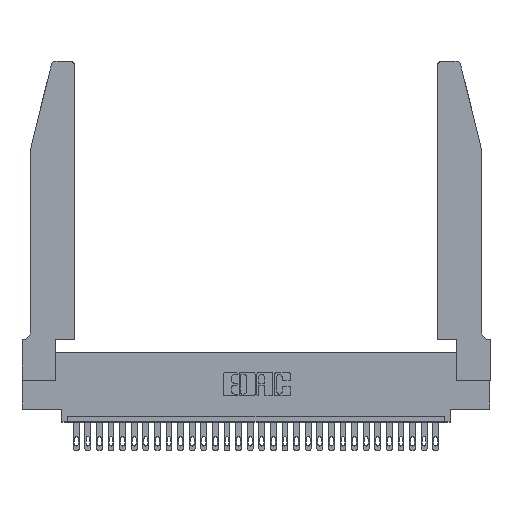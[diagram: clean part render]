
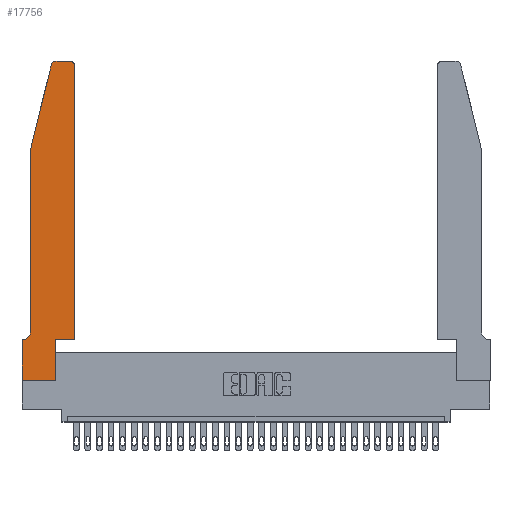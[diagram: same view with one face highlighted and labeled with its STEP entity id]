
A CAD part, top view. The second image highlights one B-rep face of the part: STEP entity #17756.
In plain terms, the highlighted planar face has unit normal (0, 0, 1).
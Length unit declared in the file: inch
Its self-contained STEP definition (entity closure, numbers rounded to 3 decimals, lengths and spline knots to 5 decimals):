
#52 = DIRECTION ( 'NONE',  ( -1., 0., 0. ) ) ;
#179 = VECTOR ( 'NONE', #19722, 39.37008 ) ;
#254 = EDGE_CURVE ( 'NONE', #11157, #16692, #16681, .T. ) ;
#274 = CARTESIAN_POINT ( 'NONE',  ( 0.4505, 0.35, 0.37 ) ) ;
#469 = ORIENTED_EDGE ( 'NONE', *, *, #24269, .T. ) ;
#920 = ORIENTED_EDGE ( 'NONE', *, *, #14897, .T. ) ;
#922 = DIRECTION ( 'NONE',  ( 1., 0., 0. ) ) ;
#1489 = LINE ( 'NONE', #13190, #11700 ) ;
#1557 = ORIENTED_EDGE ( 'NONE', *, *, #24972, .T. ) ;
#1760 = CARTESIAN_POINT ( 'NONE',  ( 0.284, 2.75, 0.37 ) ) ;
#1911 = DIRECTION ( 'NONE',  ( 0., 0., -1. ) ) ;
#2083 = CARTESIAN_POINT ( 'NONE',  ( 0.0755, 2., 0.37 ) ) ;
#3537 = CARTESIAN_POINT ( 'NONE',  ( 0., 0., 0.37 ) ) ;
#3926 = DIRECTION ( 'NONE',  ( 1., 0., 0. ) ) ;
#4260 = DIRECTION ( 'NONE',  ( -1., 0., 0. ) ) ;
#4285 = VECTOR ( 'NONE', #26465, 39.37008 ) ;
#4305 = VECTOR ( 'NONE', #22898, 39.37008 ) ;
#5096 = LINE ( 'NONE', #13707, #20082 ) ;
#5720 = CARTESIAN_POINT ( 'NONE',  ( 0.4205, 2.75, 0.37 ) ) ;
#5817 = PLANE ( 'NONE',  #21972 ) ;
#5861 = ORIENTED_EDGE ( 'NONE', *, *, #7696, .T. ) ;
#6608 = CARTESIAN_POINT ( 'NONE',  ( 0.2865, 0.35, 0.37 ) ) ;
#6617 = CARTESIAN_POINT ( 'NONE',  ( 0.0055, 0.42, 0.37 ) ) ;
#6941 = EDGE_CURVE ( 'NONE', #27220, #18902, #28655, .T. ) ;
#7156 = DIRECTION ( 'NONE',  ( 1., 0., 0. ) ) ;
#7696 = EDGE_CURVE ( 'NONE', #17560, #13418, #20553, .T. ) ;
#7703 = ORIENTED_EDGE ( 'NONE', *, *, #11444, .T. ) ;
#8068 = VERTEX_POINT ( 'NONE', #274 ) ;
#8947 = ORIENTED_EDGE ( 'NONE', *, *, #6941, .T. ) ;
#9118 = DIRECTION ( 'NONE',  ( -0.239, -0.971, 0. ) ) ;
#9748 = CARTESIAN_POINT ( 'NONE',  ( 0.2605, 2.75, 0.37 ) ) ;
#10065 = DIRECTION ( 'NONE',  ( 1., 0., 0. ) ) ;
#10258 = CARTESIAN_POINT ( 'NONE',  ( 0.4505, 0.35, 0.37 ) ) ;
#11040 = CARTESIAN_POINT ( 'NONE',  ( 0.4505, 2.72, 0.37 ) ) ;
#11157 = VERTEX_POINT ( 'NONE', #20898 ) ;
#11444 = EDGE_CURVE ( 'NONE', #12170, #21228, #24601, .T. ) ;
#11700 = VECTOR ( 'NONE', #3926, 39.37008 ) ;
#12170 = VERTEX_POINT ( 'NONE', #11040 ) ;
#12524 = VECTOR ( 'NONE', #9118, 39.37008 ) ;
#12871 = CARTESIAN_POINT ( 'NONE',  ( 0.0755, 0.42, 0.37 ) ) ;
#13190 = CARTESIAN_POINT ( 'NONE',  ( 0., 0., 0.37 ) ) ;
#13364 = ORIENTED_EDGE ( 'NONE', *, *, #19137, .T. ) ;
#13418 = VERTEX_POINT ( 'NONE', #21929 ) ;
#13707 = CARTESIAN_POINT ( 'NONE',  ( 0.0755, 2., 0.37 ) ) ;
#13737 = VERTEX_POINT ( 'NONE', #23067 ) ;
#14010 = CARTESIAN_POINT ( 'NONE',  ( 0.0755, 0.35, 0.37 ) ) ;
#14469 = FACE_OUTER_BOUND ( 'NONE', #20575, .T. ) ;
#14897 = EDGE_CURVE ( 'NONE', #13418, #27005, #5096, .T. ) ;
#15556 = VERTEX_POINT ( 'NONE', #1760 ) ;
#16206 = CARTESIAN_POINT ( 'NONE',  ( 0.4505, 0.35, 0.37 ) ) ;
#16681 = LINE ( 'NONE', #6608, #4305 ) ;
#16692 = VERTEX_POINT ( 'NONE', #29117 ) ;
#17285 = DIRECTION ( 'NONE',  ( 0., -1., 0. ) ) ;
#17389 = LINE ( 'NONE', #9748, #4285 ) ;
#17560 = VERTEX_POINT ( 'NONE', #22839 ) ;
#17756 = ADVANCED_FACE ( 'NONE', ( #14469 ), #5817, .T. ) ;
#18219 = VECTOR ( 'NONE', #52, 39.37008 ) ;
#18856 = AXIS2_PLACEMENT_3D ( 'NONE', #6617, #1911, #4260 ) ;
#18902 = VERTEX_POINT ( 'NONE', #29176 ) ;
#19137 = EDGE_CURVE ( 'NONE', #16692, #8068, #26073, .T. ) ;
#19182 = CIRCLE ( 'NONE', #19383, 0.03 ) ;
#19324 = CARTESIAN_POINT ( 'NONE',  ( 0.4205, 2.72, 0.37 ) ) ;
#19363 = EDGE_CURVE ( 'NONE', #8068, #12170, #26429, .T. ) ;
#19383 = AXIS2_PLACEMENT_3D ( 'NONE', #21710, #26424, #24180 ) ;
#19722 = DIRECTION ( 'NONE',  ( 0., 1., 0. ) ) ;
#19771 = ORIENTED_EDGE ( 'NONE', *, *, #254, .T. ) ;
#19847 = DIRECTION ( 'NONE',  ( 0., 0., 1. ) ) ;
#20082 = VECTOR ( 'NONE', #22881, 39.37008 ) ;
#20432 = LINE ( 'NONE', #14010, #18219 ) ;
#20516 = CARTESIAN_POINT ( 'NONE',  ( 0., 0.35, 0.37 ) ) ;
#20553 = LINE ( 'NONE', #2083, #12524 ) ;
#20575 = EDGE_LOOP ( 'NONE', ( #469, #1557, #5861, #920, #24617, #27003, #8947, #25958, #19771, #13364, #24503, #7703 ) ) ;
#20898 = CARTESIAN_POINT ( 'NONE',  ( 0.2865, 0., 0.37 ) ) ;
#21228 = VERTEX_POINT ( 'NONE', #5720 ) ;
#21676 = DIRECTION ( 'NONE',  ( 0., 0., 1. ) ) ;
#21710 = CARTESIAN_POINT ( 'NONE',  ( 0.284, 2.72, 0.37 ) ) ;
#21929 = CARTESIAN_POINT ( 'NONE',  ( 0.0755, 2., 0.37 ) ) ;
#21972 = AXIS2_PLACEMENT_3D ( 'NONE', #26706, #19847, #922 ) ;
#22350 = CIRCLE ( 'NONE', #18856, 0.07 ) ;
#22839 = CARTESIAN_POINT ( 'NONE',  ( 0.25487, 2.72718, 0.37 ) ) ;
#22881 = DIRECTION ( 'NONE',  ( 0., -1., 0. ) ) ;
#22898 = DIRECTION ( 'NONE',  ( 0., 1., 0. ) ) ;
#23067 = CARTESIAN_POINT ( 'NONE',  ( 0.0055, 0.35, 0.37 ) ) ;
#23725 = AXIS2_PLACEMENT_3D ( 'NONE', #19324, #21676, #10065 ) ;
#24180 = DIRECTION ( 'NONE',  ( 1., 0., 0. ) ) ;
#24269 = EDGE_CURVE ( 'NONE', #21228, #15556, #17389, .T. ) ;
#24503 = ORIENTED_EDGE ( 'NONE', *, *, #19363, .T. ) ;
#24601 = CIRCLE ( 'NONE', #23725, 0.03 ) ;
#24617 = ORIENTED_EDGE ( 'NONE', *, *, #28520, .T. ) ;
#24972 = EDGE_CURVE ( 'NONE', #15556, #17560, #19182, .T. ) ;
#25958 = ORIENTED_EDGE ( 'NONE', *, *, #29963, .T. ) ;
#26073 = LINE ( 'NONE', #16206, #28647 ) ;
#26424 = DIRECTION ( 'NONE',  ( 0., 0., 1. ) ) ;
#26429 = LINE ( 'NONE', #10258, #179 ) ;
#26465 = DIRECTION ( 'NONE',  ( -1., 0., 0. ) ) ;
#26706 = CARTESIAN_POINT ( 'NONE',  ( 0., 0.35, 0.37 ) ) ;
#27003 = ORIENTED_EDGE ( 'NONE', *, *, #30146, .T. ) ;
#27005 = VERTEX_POINT ( 'NONE', #12871 ) ;
#27220 = VERTEX_POINT ( 'NONE', #20516 ) ;
#28520 = EDGE_CURVE ( 'NONE', #27005, #13737, #22350, .T. ) ;
#28647 = VECTOR ( 'NONE', #7156, 39.37008 ) ;
#28655 = LINE ( 'NONE', #3537, #29378 ) ;
#29117 = CARTESIAN_POINT ( 'NONE',  ( 0.2865, 0.35, 0.37 ) ) ;
#29176 = CARTESIAN_POINT ( 'NONE',  ( 0., 0., 0.37 ) ) ;
#29378 = VECTOR ( 'NONE', #17285, 39.37008 ) ;
#29963 = EDGE_CURVE ( 'NONE', #18902, #11157, #1489, .T. ) ;
#30146 = EDGE_CURVE ( 'NONE', #13737, #27220, #20432, .T. ) ;
